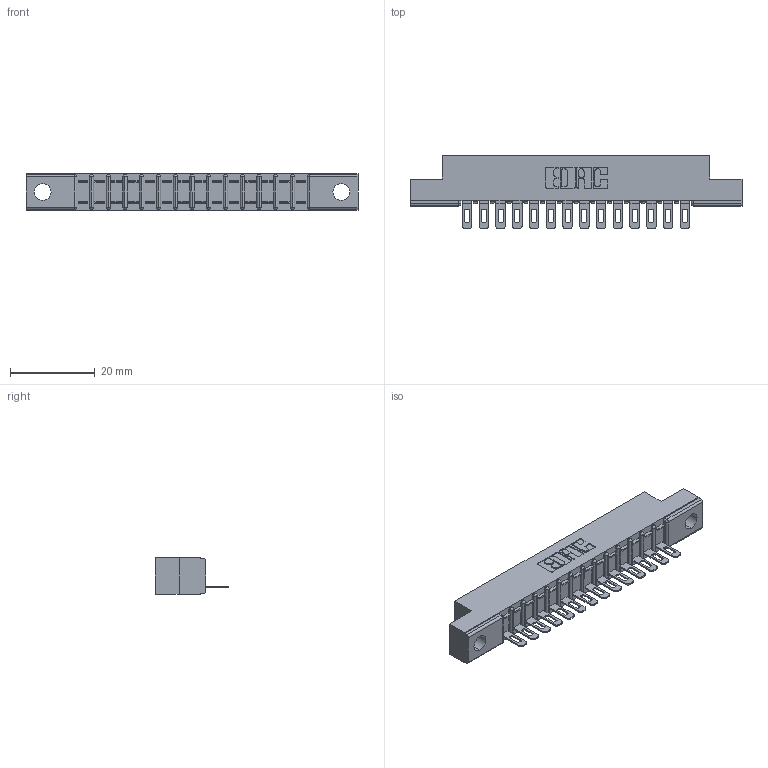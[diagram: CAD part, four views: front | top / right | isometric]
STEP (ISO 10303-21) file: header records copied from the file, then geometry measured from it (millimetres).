
FILE_DESCRIPTION (( 'STEP AP203' ), '1' );
FILE_NAME ('357-014-501-104.STEP', '2018-08-07T23:44:54', ( '' ), ( '' ), 'SwSTEP 2.0', 'SolidWorks 2016', '' );
FILE_SCHEMA (( 'CONFIG_CONTROL_DESIGN' ));
Length unit declared in the file: inch
Products named in the file (3): 307 Part_.156 Dia Mounting Holes; 307-290-002_501; 357-014-501-104
Assembly tree (15 placements, depth 2):
  357-014-501-104
    307 Part_.156 Dia Mounting Holes
    307-290-002_501  x14
Bounding box: 78.49 x 17.42 x 8.71 mm (x, y, z)
Volume: 5083.6 mm3; surface area: 8786.3 mm2
Topology: 15 solids, 15 shells, 1211 faces, 3691 edges, 2418 vertices
Faces by surface type: plane 700, cylinder 481, sphere 30
Entity records: 16666 total; most frequent: CARTESIAN_POINT 2810, ORIENTED_EDGE 2798, DIRECTION 2739, EDGE_CURVE 1399, VECTOR 1061, LINE 1061, VERTEX_POINT 910, AXIS2_PLACEMENT_3D 839
